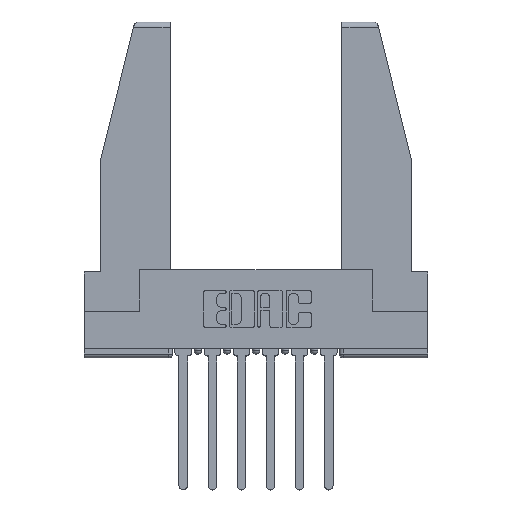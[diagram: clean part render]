
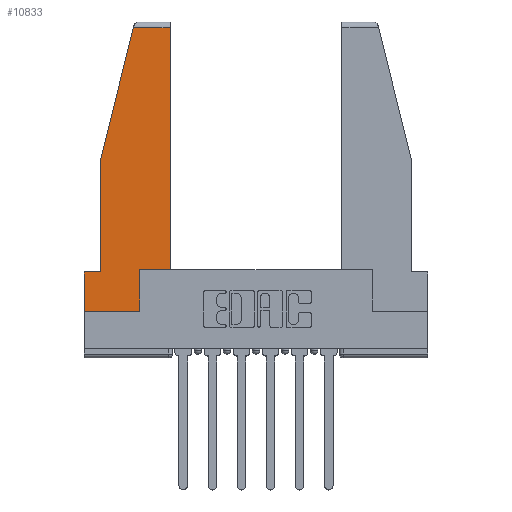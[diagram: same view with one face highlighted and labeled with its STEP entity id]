
A CAD part, top view. The second image highlights one B-rep face of the part: STEP entity #10833.
In plain terms, the highlighted planar face has unit normal (0, 0, 1).
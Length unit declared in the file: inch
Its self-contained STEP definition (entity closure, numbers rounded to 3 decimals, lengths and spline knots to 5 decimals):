
#31 = ORIENTED_EDGE ( 'NONE', *, *, #5258, .T. ) ;
#96 = CARTESIAN_POINT ( 'NONE',  ( 0., 0.21, 0. ) ) ;
#240 = CARTESIAN_POINT ( 'NONE',  ( 0., 0., 0. ) ) ;
#323 = VERTEX_POINT ( 'NONE', #8989 ) ;
#344 = ORIENTED_EDGE ( 'NONE', *, *, #7592, .T. ) ;
#482 = PLANE ( 'NONE',  #4821 ) ;
#564 = EDGE_CURVE ( 'NONE', #5219, #7845, #11619, .T. ) ;
#618 = VERTEX_POINT ( 'NONE', #1185 ) ;
#1185 = CARTESIAN_POINT ( 'NONE',  ( 0.297, 0.223, 0. ) ) ;
#1214 = VECTOR ( 'NONE', #9352, 39.37008 ) ;
#1241 = LINE ( 'NONE', #2799, #6541 ) ;
#1442 = CARTESIAN_POINT ( 'NONE',  ( 0., 0., 0. ) ) ;
#1518 = EDGE_CURVE ( 'NONE', #11171, #5219, #9241, .T. ) ;
#1667 = VECTOR ( 'NONE', #5681, 39.37008 ) ;
#1795 = EDGE_CURVE ( 'NONE', #7845, #618, #5816, .T. ) ;
#2118 = VERTEX_POINT ( 'NONE', #4391 ) ;
#2206 = CARTESIAN_POINT ( 'NONE',  ( 0.297, 0.223, 0. ) ) ;
#2301 = ORIENTED_EDGE ( 'NONE', *, *, #564, .T. ) ;
#2439 = CARTESIAN_POINT ( 'NONE',  ( 0., 1.52, 0. ) ) ;
#2555 = CARTESIAN_POINT ( 'NONE',  ( 0., 0.21, 0. ) ) ;
#2771 = EDGE_LOOP ( 'NONE', ( #344, #3070, #31, #2788, #4596, #10533, #2301, #10557, #6749 ) ) ;
#2788 = ORIENTED_EDGE ( 'NONE', *, *, #3004, .T. ) ;
#2799 = CARTESIAN_POINT ( 'NONE',  ( 0.086, 0.8, 0. ) ) ;
#3004 = EDGE_CURVE ( 'NONE', #5418, #323, #1241, .T. ) ;
#3037 = VECTOR ( 'NONE', #3489, 39.37008 ) ;
#3070 = ORIENTED_EDGE ( 'NONE', *, *, #10743, .T. ) ;
#3317 = DIRECTION ( 'NONE',  ( -1., 0., 0. ) ) ;
#3489 = DIRECTION ( 'NONE',  ( 0., -1., 0. ) ) ;
#3562 = DIRECTION ( 'NONE',  ( 0., 0., 1. ) ) ;
#3775 = CARTESIAN_POINT ( 'NONE',  ( 0.461, 0.223, 0. ) ) ;
#3939 = DIRECTION ( 'NONE',  ( 1., 0., 0. ) ) ;
#3984 = LINE ( 'NONE', #5811, #1214 ) ;
#4364 = CARTESIAN_POINT ( 'NONE',  ( 0.297, 0., 0. ) ) ;
#4391 = CARTESIAN_POINT ( 'NONE',  ( 0.461, 1.52, 0. ) ) ;
#4596 = ORIENTED_EDGE ( 'NONE', *, *, #5666, .T. ) ;
#4776 = CARTESIAN_POINT ( 'NONE',  ( 0., 0.21, 0. ) ) ;
#4821 = AXIS2_PLACEMENT_3D ( 'NONE', #1442, #3562, #6235 ) ;
#4926 = VERTEX_POINT ( 'NONE', #3775 ) ;
#5219 = VERTEX_POINT ( 'NONE', #10390 ) ;
#5258 = EDGE_CURVE ( 'NONE', #8777, #5418, #3984, .T. ) ;
#5382 = VECTOR ( 'NONE', #10464, 39.37008 ) ;
#5418 = VERTEX_POINT ( 'NONE', #11892 ) ;
#5666 = EDGE_CURVE ( 'NONE', #323, #11171, #10790, .T. ) ;
#5681 = DIRECTION ( 'NONE',  ( -1., 0., 0. ) ) ;
#5811 = CARTESIAN_POINT ( 'NONE',  ( 0.271, 1.55, 0. ) ) ;
#5816 = LINE ( 'NONE', #11499, #5382 ) ;
#5847 = CARTESIAN_POINT ( 'NONE',  ( 0.461, 0.223, 0. ) ) ;
#6235 = DIRECTION ( 'NONE',  ( 1., 0., 0. ) ) ;
#6510 = LINE ( 'NONE', #5847, #8853 ) ;
#6541 = VECTOR ( 'NONE', #9659, 39.37008 ) ;
#6749 = ORIENTED_EDGE ( 'NONE', *, *, #9940, .T. ) ;
#7214 = LINE ( 'NONE', #2206, #8810 ) ;
#7592 = EDGE_CURVE ( 'NONE', #4926, #2118, #6510, .T. ) ;
#7841 = DIRECTION ( 'NONE',  ( 1., 0., 0. ) ) ;
#7845 = VERTEX_POINT ( 'NONE', #4364 ) ;
#8641 = VECTOR ( 'NONE', #3317, 39.37008 ) ;
#8777 = VERTEX_POINT ( 'NONE', #8866 ) ;
#8810 = VECTOR ( 'NONE', #3939, 39.37008 ) ;
#8853 = VECTOR ( 'NONE', #10474, 39.37008 ) ;
#8866 = CARTESIAN_POINT ( 'NONE',  ( 0.2636, 1.52, 0. ) ) ;
#8989 = CARTESIAN_POINT ( 'NONE',  ( 0.086, 0.21, 0. ) ) ;
#9241 = LINE ( 'NONE', #2555, #3037 ) ;
#9352 = DIRECTION ( 'NONE',  ( -0.239, -0.971, 0. ) ) ;
#9659 = DIRECTION ( 'NONE',  ( 0., -1., 0. ) ) ;
#9940 = EDGE_CURVE ( 'NONE', #618, #4926, #7214, .T. ) ;
#10390 = CARTESIAN_POINT ( 'NONE',  ( 0., 0., 0. ) ) ;
#10464 = DIRECTION ( 'NONE',  ( 0., 1., 0. ) ) ;
#10474 = DIRECTION ( 'NONE',  ( 0., 1., 0. ) ) ;
#10533 = ORIENTED_EDGE ( 'NONE', *, *, #1518, .T. ) ;
#10557 = ORIENTED_EDGE ( 'NONE', *, *, #1795, .T. ) ;
#10743 = EDGE_CURVE ( 'NONE', #2118, #8777, #11912, .T. ) ;
#10790 = LINE ( 'NONE', #96, #1667 ) ;
#10833 = ADVANCED_FACE ( 'NONE', ( #11763 ), #482, .T. ) ;
#11038 = VECTOR ( 'NONE', #7841, 39.37008 ) ;
#11171 = VERTEX_POINT ( 'NONE', #4776 ) ;
#11499 = CARTESIAN_POINT ( 'NONE',  ( 0.297, 0., 0. ) ) ;
#11619 = LINE ( 'NONE', #240, #11038 ) ;
#11763 = FACE_OUTER_BOUND ( 'NONE', #2771, .T. ) ;
#11892 = CARTESIAN_POINT ( 'NONE',  ( 0.086, 0.8, 0. ) ) ;
#11912 = LINE ( 'NONE', #2439, #8641 ) ;
